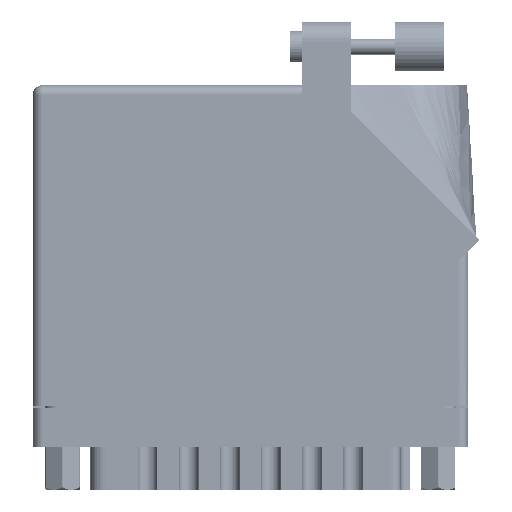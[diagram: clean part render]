
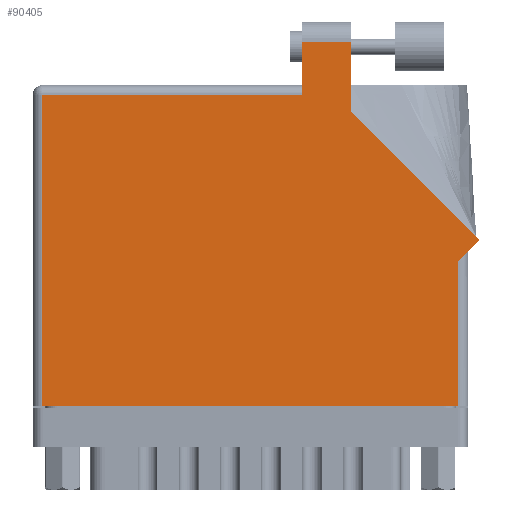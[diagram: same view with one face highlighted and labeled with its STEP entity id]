
A CAD part, front view. The second image highlights one B-rep face of the part: STEP entity #90405.
In plain terms, the highlighted face is planar.
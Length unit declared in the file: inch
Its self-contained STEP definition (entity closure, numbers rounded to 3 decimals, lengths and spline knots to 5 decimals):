
#65 = VERTEX_POINT ( 'NONE', #22691 ) ;
#396 = VECTOR ( 'NONE', #43155, 39.37008 ) ;
#1688 = DIRECTION ( 'NONE',  ( 0.707, 0.707, 0. ) ) ;
#2232 = FACE_OUTER_BOUND ( 'NONE', #66427, .T. ) ;
#2417 = VECTOR ( 'NONE', #66952, 39.37008 ) ;
#4356 = CARTESIAN_POINT ( 'NONE',  ( 2.012, 1.86442, 0. ) ) ;
#4878 = DIRECTION ( 'NONE',  ( 0., 0., -1. ) ) ;
#7533 = VERTEX_POINT ( 'NONE', #65755 ) ;
#8896 = ORIENTED_EDGE ( 'NONE', *, *, #34397, .T. ) ;
#10153 = LINE ( 'NONE', #23413, #94588 ) ;
#10522 = VERTEX_POINT ( 'NONE', #88998 ) ;
#12068 = ORIENTED_EDGE ( 'NONE', *, *, #63103, .T. ) ;
#12095 = CARTESIAN_POINT ( 'NONE',  ( 0.062, 1.968, 0. ) ) ;
#12134 = LINE ( 'NONE', #25402, #67111 ) ;
#12696 = VECTOR ( 'NONE', #87630, 39.37008 ) ;
#14138 = EDGE_CURVE ( 'NONE', #43934, #7533, #10153, .T. ) ;
#18321 = CARTESIAN_POINT ( 'NONE',  ( 1.705, 2.03, 0. ) ) ;
#22691 = CARTESIAN_POINT ( 'NONE',  ( 1.705, 1.968, 0. ) ) ;
#23413 = CARTESIAN_POINT ( 'NONE',  ( 0., 0., 0. ) ) ;
#25223 = CARTESIAN_POINT ( 'NONE',  ( 2.693, 0.918, 0. ) ) ;
#25402 = CARTESIAN_POINT ( 'NONE',  ( 2.755, 0.98, 0. ) ) ;
#26829 = LINE ( 'NONE', #95703, #104950 ) ;
#27480 = EDGE_CURVE ( 'NONE', #65, #32020, #50524, .T. ) ;
#28030 = ORIENTED_EDGE ( 'NONE', *, *, #27480, .T. ) ;
#28997 = ORIENTED_EDGE ( 'NONE', *, *, #103022, .T. ) ;
#30363 = LINE ( 'NONE', #53647, #92998 ) ;
#31145 = CARTESIAN_POINT ( 'NONE',  ( 1.705, 2.305, 0. ) ) ;
#32020 = VERTEX_POINT ( 'NONE', #12095 ) ;
#34257 = DIRECTION ( 'NONE',  ( -1., 0., 0. ) ) ;
#34397 = EDGE_CURVE ( 'NONE', #7533, #62064, #44008, .T. ) ;
#34441 = ORIENTED_EDGE ( 'NONE', *, *, #47879, .T. ) ;
#38187 = CARTESIAN_POINT ( 'NONE',  ( 0., 2.03, 0. ) ) ;
#40130 = VERTEX_POINT ( 'NONE', #49616 ) ;
#41474 = LINE ( 'NONE', #46967, #63191 ) ;
#43155 = DIRECTION ( 'NONE',  ( 0., 1., 0. ) ) ;
#43176 = CARTESIAN_POINT ( 'NONE',  ( 0., 1.968, 0. ) ) ;
#43934 = VERTEX_POINT ( 'NONE', #58075 ) ;
#44008 = LINE ( 'NONE', #67447, #396 ) ;
#44351 = VERTEX_POINT ( 'NONE', #95204 ) ;
#44920 = EDGE_CURVE ( 'NONE', #40130, #10522, #101407, .T. ) ;
#46967 = CARTESIAN_POINT ( 'NONE',  ( 2.82571, 1.05071, 0. ) ) ;
#47879 = EDGE_CURVE ( 'NONE', #44351, #105343, #41474, .T. ) ;
#48378 = ORIENTED_EDGE ( 'NONE', *, *, #60616, .T. ) ;
#49616 = CARTESIAN_POINT ( 'NONE',  ( 2.012, 2.305, 0. ) ) ;
#50524 = LINE ( 'NONE', #43176, #97805 ) ;
#51401 = EDGE_CURVE ( 'NONE', #32020, #43934, #26829, .T. ) ;
#53559 = DIRECTION ( 'NONE',  ( 0., -1., 0. ) ) ;
#53647 = CARTESIAN_POINT ( 'NONE',  ( 2.012, 1.86442, 0. ) ) ;
#55888 = ORIENTED_EDGE ( 'NONE', *, *, #44920, .T. ) ;
#55907 = ORIENTED_EDGE ( 'NONE', *, *, #51401, .T. ) ;
#58075 = CARTESIAN_POINT ( 'NONE',  ( 0.062, 0., 0. ) ) ;
#60616 = EDGE_CURVE ( 'NONE', #10522, #65, #77991, .T. ) ;
#62064 = VERTEX_POINT ( 'NONE', #25223 ) ;
#63103 = EDGE_CURVE ( 'NONE', #105343, #40130, #30363, .T. ) ;
#63191 = VECTOR ( 'NONE', #78387, 39.37008 ) ;
#65755 = CARTESIAN_POINT ( 'NONE',  ( 2.693, 0., 0. ) ) ;
#66427 = EDGE_LOOP ( 'NONE', ( #12068, #55888, #48378, #28030, #55907, #102719, #8896, #28997, #34441 ) ) ;
#66952 = DIRECTION ( 'NONE',  ( 0., -1., 0. ) ) ;
#67111 = VECTOR ( 'NONE', #1688, 39.37008 ) ;
#67447 = CARTESIAN_POINT ( 'NONE',  ( 2.693, 0.98, 0. ) ) ;
#72353 = DIRECTION ( 'NONE',  ( 1., 0., 0. ) ) ;
#77991 = LINE ( 'NONE', #18321, #2417 ) ;
#78387 = DIRECTION ( 'NONE',  ( -0.707, 0.707, 0. ) ) ;
#78542 = PLANE ( 'NONE',  #101772 ) ;
#87630 = DIRECTION ( 'NONE',  ( -1., 0., 0. ) ) ;
#88998 = CARTESIAN_POINT ( 'NONE',  ( 1.705, 2.305, 0. ) ) ;
#90405 = ADVANCED_FACE ( 'NONE', ( #2232 ), #78542, .F. ) ;
#92998 = VECTOR ( 'NONE', #94369, 39.37008 ) ;
#94369 = DIRECTION ( 'NONE',  ( 0., 1., 0. ) ) ;
#94588 = VECTOR ( 'NONE', #72353, 39.37008 ) ;
#95204 = CARTESIAN_POINT ( 'NONE',  ( 2.82571, 1.05071, 0. ) ) ;
#95363 = DIRECTION ( 'NONE',  ( -1., 0., 0. ) ) ;
#95703 = CARTESIAN_POINT ( 'NONE',  ( 0.062, 0., 0. ) ) ;
#97805 = VECTOR ( 'NONE', #34257, 39.37008 ) ;
#101407 = LINE ( 'NONE', #31145, #12696 ) ;
#101772 = AXIS2_PLACEMENT_3D ( 'NONE', #38187, #4878, #95363 ) ;
#102719 = ORIENTED_EDGE ( 'NONE', *, *, #14138, .T. ) ;
#103022 = EDGE_CURVE ( 'NONE', #62064, #44351, #12134, .T. ) ;
#104950 = VECTOR ( 'NONE', #53559, 39.37008 ) ;
#105343 = VERTEX_POINT ( 'NONE', #4356 ) ;
